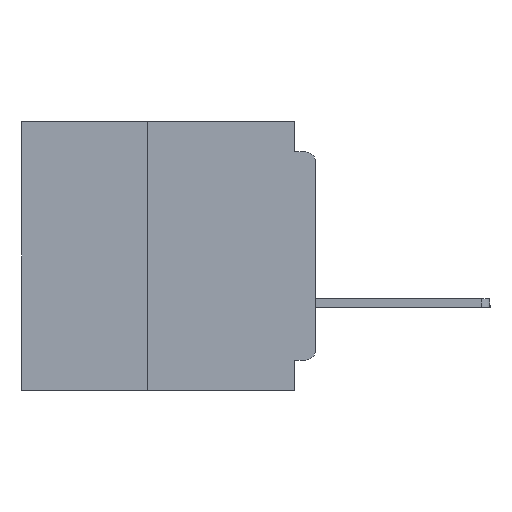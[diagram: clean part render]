
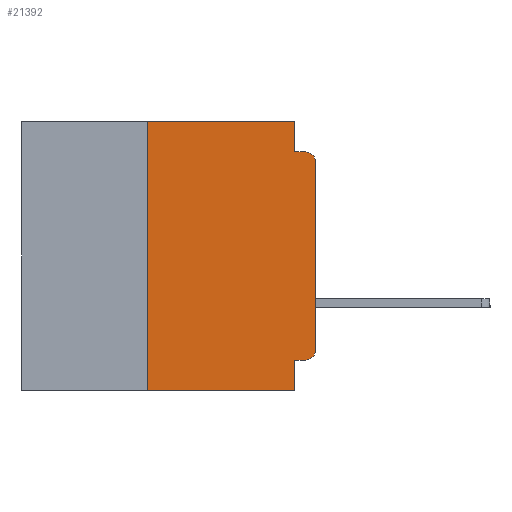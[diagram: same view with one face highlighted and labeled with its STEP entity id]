
A CAD part, left-side view. The second image highlights one B-rep face of the part: STEP entity #21392.
In plain terms, the highlighted planar face has unit normal (-1, 0, 0).
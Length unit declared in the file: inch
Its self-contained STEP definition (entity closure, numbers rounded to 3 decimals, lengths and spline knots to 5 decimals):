
#1881 = ORIENTED_EDGE ( 'NONE', *, *, #49718, .T. ) ;
#2068 = LINE ( 'NONE', #39026, #16186 ) ;
#2459 = CARTESIAN_POINT ( 'NONE',  ( 0., 0.437, -0.4 ) ) ;
#2904 = VERTEX_POINT ( 'NONE', #10195 ) ;
#3924 = CARTESIAN_POINT ( 'NONE',  ( 0., 0.031, 0. ) ) ;
#4033 = ORIENTED_EDGE ( 'NONE', *, *, #68207, .T. ) ;
#4749 = CARTESIAN_POINT ( 'NONE',  ( 0., 0.031, -0.045 ) ) ;
#4768 = EDGE_CURVE ( 'NONE', #8710, #25435, #41983, .T. ) ;
#6350 = ORIENTED_EDGE ( 'NONE', *, *, #64386, .F. ) ;
#6529 = EDGE_CURVE ( 'NONE', #2904, #25511, #41931, .T. ) ;
#6679 = EDGE_CURVE ( 'NONE', #66320, #43352, #2068, .T. ) ;
#7224 = DIRECTION ( 'NONE',  ( 0., 1., 0. ) ) ;
#8057 = LINE ( 'NONE', #3924, #61126 ) ;
#8346 = AXIS2_PLACEMENT_3D ( 'NONE', #28449, #44389, #12614 ) ;
#8710 = VERTEX_POINT ( 'NONE', #18198 ) ;
#8981 = VECTOR ( 'NONE', #53727, 39.37008 ) ;
#9209 = VECTOR ( 'NONE', #63195, 39.37008 ) ;
#9844 = EDGE_CURVE ( 'NONE', #8710, #38310, #20872, .T. ) ;
#10195 = CARTESIAN_POINT ( 'NONE',  ( 0., 0., -0.34 ) ) ;
#11721 = ORIENTED_EDGE ( 'NONE', *, *, #9844, .T. ) ;
#11918 = CARTESIAN_POINT ( 'NONE',  ( 0., 0.015, -0.34 ) ) ;
#12589 = ORIENTED_EDGE ( 'NONE', *, *, #6679, .F. ) ;
#12614 = DIRECTION ( 'NONE',  ( 0., 0., -1. ) ) ;
#13693 = VECTOR ( 'NONE', #42751, 39.37008 ) ;
#16186 = VECTOR ( 'NONE', #7224, 39.37008 ) ;
#16332 = CARTESIAN_POINT ( 'NONE',  ( 0., 0., 0. ) ) ;
#17197 = DIRECTION ( 'NONE',  ( 0., 0., 1. ) ) ;
#17309 = DIRECTION ( 'NONE',  ( 0., 0., -1. ) ) ;
#18198 = CARTESIAN_POINT ( 'NONE',  ( 0., 0.25, -0.4 ) ) ;
#18371 = AXIS2_PLACEMENT_3D ( 'NONE', #11918, #48979, #17309 ) ;
#19963 = FACE_OUTER_BOUND ( 'NONE', #40526, .T. ) ;
#20872 = LINE ( 'NONE', #2459, #33274 ) ;
#20976 = AXIS2_PLACEMENT_3D ( 'NONE', #28804, #65776, #34126 ) ;
#21104 = CARTESIAN_POINT ( 'NONE',  ( 0., 0.031, -0.4 ) ) ;
#21392 = ADVANCED_FACE ( 'NONE', ( #19963 ), #54770, .F. ) ;
#22835 = CARTESIAN_POINT ( 'NONE',  ( 0., 0.25, 0. ) ) ;
#23185 = LINE ( 'NONE', #64151, #8981 ) ;
#24329 = LINE ( 'NONE', #58237, #64833 ) ;
#25435 = VERTEX_POINT ( 'NONE', #22835 ) ;
#25511 = VERTEX_POINT ( 'NONE', #45480 ) ;
#26575 = VERTEX_POINT ( 'NONE', #48242 ) ;
#28412 = CIRCLE ( 'NONE', #18371, 0.015 ) ;
#28449 = CARTESIAN_POINT ( 'NONE',  ( 0., 0.437, 0. ) ) ;
#28804 = CARTESIAN_POINT ( 'NONE',  ( 0., 0.015, -0.06 ) ) ;
#31155 = VERTEX_POINT ( 'NONE', #4749 ) ;
#31468 = EDGE_CURVE ( 'NONE', #43352, #38310, #23185, .T. ) ;
#33274 = VECTOR ( 'NONE', #50205, 39.37008 ) ;
#34126 = DIRECTION ( 'NONE',  ( 0., 0., -1. ) ) ;
#35752 = DIRECTION ( 'NONE',  ( 0., 0., -1. ) ) ;
#37178 = DIRECTION ( 'NONE',  ( 0., -1., 0. ) ) ;
#38310 = VERTEX_POINT ( 'NONE', #21104 ) ;
#38334 = VERTEX_POINT ( 'NONE', #42592 ) ;
#39026 = CARTESIAN_POINT ( 'NONE',  ( 0., 0., -0.355 ) ) ;
#39135 = LINE ( 'NONE', #57866, #9209 ) ;
#39448 = EDGE_CURVE ( 'NONE', #26575, #31155, #8057, .T. ) ;
#40526 = EDGE_LOOP ( 'NONE', ( #59350, #1881, #68003, #48945, #6350, #65085, #11721, #66202, #12589, #4033 ) ) ;
#41300 = CARTESIAN_POINT ( 'NONE',  ( 0., 0.031, -0.355 ) ) ;
#41931 = LINE ( 'NONE', #16332, #13693 ) ;
#41983 = LINE ( 'NONE', #48863, #43650 ) ;
#42592 = CARTESIAN_POINT ( 'NONE',  ( 0., 0.015, -0.045 ) ) ;
#42751 = DIRECTION ( 'NONE',  ( 0., 0., 1. ) ) ;
#43352 = VERTEX_POINT ( 'NONE', #41300 ) ;
#43650 = VECTOR ( 'NONE', #17197, 39.37008 ) ;
#44389 = DIRECTION ( 'NONE',  ( 1., 0., 0. ) ) ;
#45480 = CARTESIAN_POINT ( 'NONE',  ( 0., 0., -0.06 ) ) ;
#47857 = CARTESIAN_POINT ( 'NONE',  ( 0., 0.015, -0.355 ) ) ;
#48242 = CARTESIAN_POINT ( 'NONE',  ( 0., 0.031, 0. ) ) ;
#48863 = CARTESIAN_POINT ( 'NONE',  ( 0., 0.25, -0.4 ) ) ;
#48945 = ORIENTED_EDGE ( 'NONE', *, *, #39448, .F. ) ;
#48979 = DIRECTION ( 'NONE',  ( -1., 0., 0. ) ) ;
#49718 = EDGE_CURVE ( 'NONE', #25511, #38334, #58074, .T. ) ;
#50084 = EDGE_CURVE ( 'NONE', #31155, #38334, #39135, .T. ) ;
#50205 = DIRECTION ( 'NONE',  ( 0., -1., 0. ) ) ;
#53727 = DIRECTION ( 'NONE',  ( 0., 0., -1. ) ) ;
#54770 = PLANE ( 'NONE',  #8346 ) ;
#57866 = CARTESIAN_POINT ( 'NONE',  ( 0., 0., -0.045 ) ) ;
#58074 = CIRCLE ( 'NONE', #20976, 0.015 ) ;
#58237 = CARTESIAN_POINT ( 'NONE',  ( 0., 0.437, 0. ) ) ;
#59350 = ORIENTED_EDGE ( 'NONE', *, *, #6529, .T. ) ;
#61126 = VECTOR ( 'NONE', #35752, 39.37008 ) ;
#63195 = DIRECTION ( 'NONE',  ( 0., -1., 0. ) ) ;
#64151 = CARTESIAN_POINT ( 'NONE',  ( 0., 0.031, -0.4 ) ) ;
#64386 = EDGE_CURVE ( 'NONE', #25435, #26575, #24329, .T. ) ;
#64833 = VECTOR ( 'NONE', #37178, 39.37008 ) ;
#65085 = ORIENTED_EDGE ( 'NONE', *, *, #4768, .F. ) ;
#65776 = DIRECTION ( 'NONE',  ( -1., 0., 0. ) ) ;
#66202 = ORIENTED_EDGE ( 'NONE', *, *, #31468, .F. ) ;
#66320 = VERTEX_POINT ( 'NONE', #47857 ) ;
#68003 = ORIENTED_EDGE ( 'NONE', *, *, #50084, .F. ) ;
#68207 = EDGE_CURVE ( 'NONE', #66320, #2904, #28412, .T. ) ;
